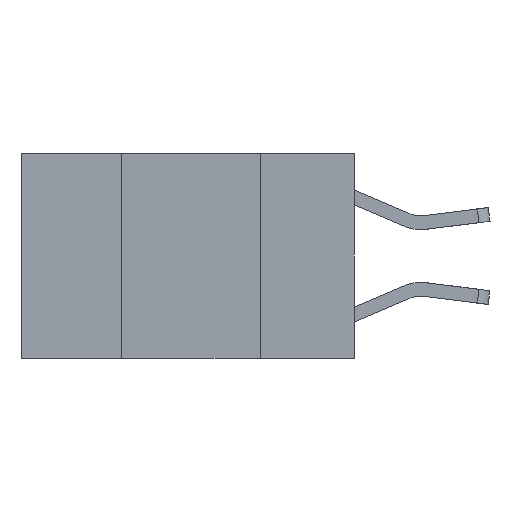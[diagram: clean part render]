
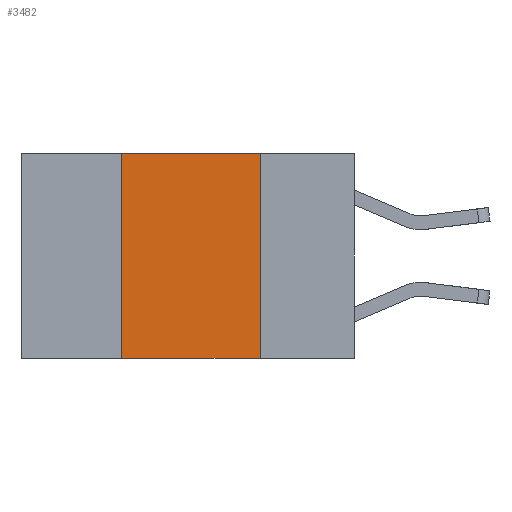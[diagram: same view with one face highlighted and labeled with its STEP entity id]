
A CAD part, left-side view. The second image highlights one B-rep face of the part: STEP entity #3482.
In plain terms, the highlighted planar face has unit normal (-1, 0, 0).
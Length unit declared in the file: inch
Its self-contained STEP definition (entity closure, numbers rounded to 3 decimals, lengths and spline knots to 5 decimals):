
#35 = VECTOR ( 'NONE', #3784, 39.37008 ) ;
#66 = FACE_OUTER_BOUND ( 'NONE', #9822, .T. ) ;
#173 = LINE ( 'NONE', #5420, #4305 ) ;
#988 = VERTEX_POINT ( 'NONE', #3703 ) ;
#1952 = VERTEX_POINT ( 'NONE', #10304 ) ;
#2969 = DIRECTION ( 'NONE',  ( 0., 0., 1. ) ) ;
#3389 = PLANE ( 'NONE',  #4671 ) ;
#3397 = VERTEX_POINT ( 'NONE', #9205 ) ;
#3482 = ADVANCED_FACE ( 'NONE', ( #66 ), #3389, .F. ) ;
#3703 = CARTESIAN_POINT ( 'NONE',  ( 0., 0.42, 0. ) ) ;
#3784 = DIRECTION ( 'NONE',  ( 0., -1., 0. ) ) ;
#4305 = VECTOR ( 'NONE', #6261, 39.37008 ) ;
#4430 = LINE ( 'NONE', #7194, #10445 ) ;
#4671 = AXIS2_PLACEMENT_3D ( 'NONE', #9304, #10014, #5089 ) ;
#4873 = LINE ( 'NONE', #6622, #9131 ) ;
#5089 = DIRECTION ( 'NONE',  ( 0., 0., -1. ) ) ;
#5147 = EDGE_CURVE ( 'NONE', #8664, #1952, #6974, .T. ) ;
#5154 = EDGE_CURVE ( 'NONE', #8664, #988, #4430, .T. ) ;
#5420 = CARTESIAN_POINT ( 'NONE',  ( 0., 0.6, 0. ) ) ;
#6261 = DIRECTION ( 'NONE',  ( 0., -1., 0. ) ) ;
#6432 = ORIENTED_EDGE ( 'NONE', *, *, #7725, .F. ) ;
#6469 = ORIENTED_EDGE ( 'NONE', *, *, #8429, .F. ) ;
#6479 = ORIENTED_EDGE ( 'NONE', *, *, #5154, .F. ) ;
#6546 = ORIENTED_EDGE ( 'NONE', *, *, #5147, .T. ) ;
#6622 = CARTESIAN_POINT ( 'NONE',  ( 0., 0.17, 0. ) ) ;
#6974 = LINE ( 'NONE', #8900, #35 ) ;
#7194 = CARTESIAN_POINT ( 'NONE',  ( 0., 0.42, 0. ) ) ;
#7466 = DIRECTION ( 'NONE',  ( 0., 0., -1. ) ) ;
#7725 = EDGE_CURVE ( 'NONE', #3397, #1952, #4873, .T. ) ;
#8332 = CARTESIAN_POINT ( 'NONE',  ( 0., 0.42, -0.37 ) ) ;
#8429 = EDGE_CURVE ( 'NONE', #988, #3397, #173, .T. ) ;
#8664 = VERTEX_POINT ( 'NONE', #8332 ) ;
#8900 = CARTESIAN_POINT ( 'NONE',  ( 0., 0.6, -0.37 ) ) ;
#9131 = VECTOR ( 'NONE', #7466, 39.37008 ) ;
#9205 = CARTESIAN_POINT ( 'NONE',  ( 0., 0.17, 0. ) ) ;
#9304 = CARTESIAN_POINT ( 'NONE',  ( 0., 0.6, 0. ) ) ;
#9822 = EDGE_LOOP ( 'NONE', ( #6432, #6469, #6479, #6546 ) ) ;
#10014 = DIRECTION ( 'NONE',  ( 1., 0., 0. ) ) ;
#10304 = CARTESIAN_POINT ( 'NONE',  ( 0., 0.17, -0.37 ) ) ;
#10445 = VECTOR ( 'NONE', #2969, 39.37008 ) ;
